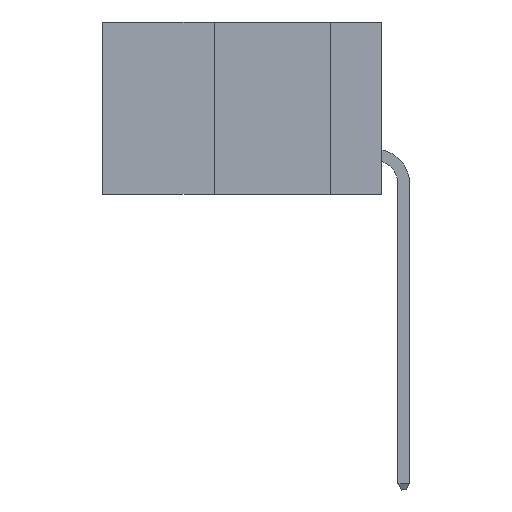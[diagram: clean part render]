
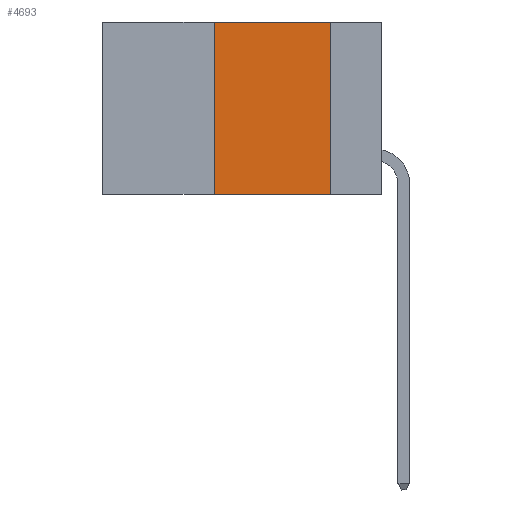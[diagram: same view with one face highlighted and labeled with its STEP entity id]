
A CAD part, left-side view. The second image highlights one B-rep face of the part: STEP entity #4693.
In plain terms, the highlighted planar face has unit normal (-1, 0, 0).
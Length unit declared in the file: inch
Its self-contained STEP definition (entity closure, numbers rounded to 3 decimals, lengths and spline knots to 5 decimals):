
#990 = DIRECTION ( 'NONE',  ( 0., -1., 0. ) ) ;
#2646 = ORIENTED_EDGE ( 'NONE', *, *, #9116, .F. ) ;
#2854 = CARTESIAN_POINT ( 'NONE',  ( 0., 0.36, 0. ) ) ;
#3724 = CARTESIAN_POINT ( 'NONE',  ( 0., 0.11, 0. ) ) ;
#3765 = ORIENTED_EDGE ( 'NONE', *, *, #28670, .F. ) ;
#4429 = EDGE_CURVE ( 'NONE', #25906, #7540, #4694, .T. ) ;
#4693 = ADVANCED_FACE ( 'NONE', ( #26225 ), #28857, .F. ) ;
#4694 = LINE ( 'NONE', #8490, #27981 ) ;
#5357 = VERTEX_POINT ( 'NONE', #10588 ) ;
#7206 = EDGE_CURVE ( 'NONE', #10181, #5357, #11956, .T. ) ;
#7540 = VERTEX_POINT ( 'NONE', #3724 ) ;
#8014 = LINE ( 'NONE', #8989, #25269 ) ;
#8490 = CARTESIAN_POINT ( 'NONE',  ( 0., 0.6, 0. ) ) ;
#8943 = LINE ( 'NONE', #22705, #18859 ) ;
#8989 = CARTESIAN_POINT ( 'NONE',  ( 0., 0.36, 0. ) ) ;
#9116 = EDGE_CURVE ( 'NONE', #7540, #5357, #8943, .T. ) ;
#10181 = VERTEX_POINT ( 'NONE', #20483 ) ;
#10459 = DIRECTION ( 'NONE',  ( 1., 0., 0. ) ) ;
#10588 = CARTESIAN_POINT ( 'NONE',  ( 0., 0.11, -0.37 ) ) ;
#11241 = VECTOR ( 'NONE', #27405, 39.37008 ) ;
#11325 = DIRECTION ( 'NONE',  ( 0., 0., 1. ) ) ;
#11956 = LINE ( 'NONE', #15836, #11241 ) ;
#13676 = CARTESIAN_POINT ( 'NONE',  ( 0., 0.6, 0. ) ) ;
#14868 = ORIENTED_EDGE ( 'NONE', *, *, #4429, .F. ) ;
#15388 = AXIS2_PLACEMENT_3D ( 'NONE', #13676, #10459, #25949 ) ;
#15836 = CARTESIAN_POINT ( 'NONE',  ( 0., 0.6, -0.37 ) ) ;
#16117 = DIRECTION ( 'NONE',  ( 0., 0., -1. ) ) ;
#18859 = VECTOR ( 'NONE', #16117, 39.37008 ) ;
#19399 = ORIENTED_EDGE ( 'NONE', *, *, #7206, .T. ) ;
#20483 = CARTESIAN_POINT ( 'NONE',  ( 0., 0.36, -0.37 ) ) ;
#22705 = CARTESIAN_POINT ( 'NONE',  ( 0., 0.11, 0. ) ) ;
#25056 = EDGE_LOOP ( 'NONE', ( #2646, #14868, #3765, #19399 ) ) ;
#25269 = VECTOR ( 'NONE', #11325, 39.37008 ) ;
#25906 = VERTEX_POINT ( 'NONE', #2854 ) ;
#25949 = DIRECTION ( 'NONE',  ( 0., 0., -1. ) ) ;
#26225 = FACE_OUTER_BOUND ( 'NONE', #25056, .T. ) ;
#27405 = DIRECTION ( 'NONE',  ( 0., -1., 0. ) ) ;
#27981 = VECTOR ( 'NONE', #990, 39.37008 ) ;
#28670 = EDGE_CURVE ( 'NONE', #10181, #25906, #8014, .T. ) ;
#28857 = PLANE ( 'NONE',  #15388 ) ;
